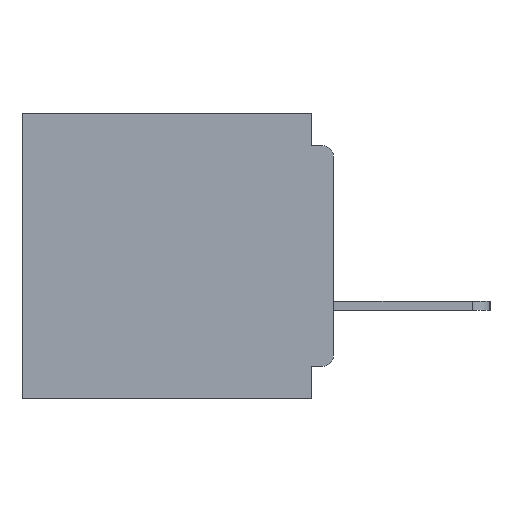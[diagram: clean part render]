
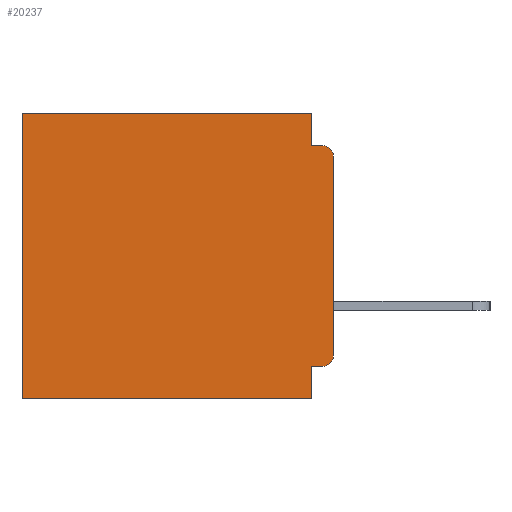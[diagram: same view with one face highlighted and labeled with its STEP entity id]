
A CAD part, left-side view. The second image highlights one B-rep face of the part: STEP entity #20237.
In plain terms, the highlighted planar face has unit normal (-1, 0, 0).
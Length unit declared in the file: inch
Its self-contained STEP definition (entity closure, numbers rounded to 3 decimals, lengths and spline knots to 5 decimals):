
#85 = EDGE_CURVE ( 'NONE', #8060, #34888, #16033, .T. ) ;
#552 = DIRECTION ( 'NONE',  ( 0., 0., -1. ) ) ;
#798 = LINE ( 'NONE', #12453, #29090 ) ;
#1566 = VECTOR ( 'NONE', #15510, 39.37008 ) ;
#2471 = LINE ( 'NONE', #6674, #1566 ) ;
#4278 = CIRCLE ( 'NONE', #12741, 0.015 ) ;
#5856 = VECTOR ( 'NONE', #15302, 39.37008 ) ;
#5936 = CARTESIAN_POINT ( 'NONE',  ( 0.3, 0.437, -0.4 ) ) ;
#6674 = CARTESIAN_POINT ( 'NONE',  ( 0.3, 0., -0.4 ) ) ;
#6757 = LINE ( 'NONE', #26754, #5856 ) ;
#6865 = EDGE_LOOP ( 'NONE', ( #32258, #36912, #10591, #34715, #27442, #28872, #13119, #13821, #22444, #24049 ) ) ;
#7541 = VECTOR ( 'NONE', #28860, 39.37008 ) ;
#8060 = VERTEX_POINT ( 'NONE', #28164 ) ;
#8603 = CARTESIAN_POINT ( 'NONE',  ( 0.3, 0., 0. ) ) ;
#8716 = VERTEX_POINT ( 'NONE', #36940 ) ;
#8830 = EDGE_CURVE ( 'NONE', #34888, #22767, #23055, .T. ) ;
#9380 = DIRECTION ( 'NONE',  ( -1., 0., 0. ) ) ;
#9565 = EDGE_CURVE ( 'NONE', #21125, #27947, #4278, .T. ) ;
#10591 = ORIENTED_EDGE ( 'NONE', *, *, #8830, .F. ) ;
#10648 = VERTEX_POINT ( 'NONE', #20290 ) ;
#11104 = AXIS2_PLACEMENT_3D ( 'NONE', #16122, #36418, #19106 ) ;
#12453 = CARTESIAN_POINT ( 'NONE',  ( 0.3, 0., -0.4 ) ) ;
#12727 = CARTESIAN_POINT ( 'NONE',  ( 0.3, 0.031, -0.045 ) ) ;
#12741 = AXIS2_PLACEMENT_3D ( 'NONE', #35406, #18072, #552 ) ;
#13091 = CARTESIAN_POINT ( 'NONE',  ( 0.3, 0.437, 0. ) ) ;
#13119 = ORIENTED_EDGE ( 'NONE', *, *, #14082, .F. ) ;
#13821 = ORIENTED_EDGE ( 'NONE', *, *, #21458, .F. ) ;
#14082 = EDGE_CURVE ( 'NONE', #23741, #10648, #798, .T. ) ;
#14494 = VECTOR ( 'NONE', #23572, 39.37008 ) ;
#15226 = AXIS2_PLACEMENT_3D ( 'NONE', #26861, #9380, #29796 ) ;
#15302 = DIRECTION ( 'NONE',  ( 0., 1., 0. ) ) ;
#15510 = DIRECTION ( 'NONE',  ( 0., 0., -1. ) ) ;
#16033 = LINE ( 'NONE', #19001, #37380 ) ;
#16122 = CARTESIAN_POINT ( 'NONE',  ( 0.3, 0., -0.4 ) ) ;
#18072 = DIRECTION ( 'NONE',  ( -1., 0., 0. ) ) ;
#18579 = CARTESIAN_POINT ( 'NONE',  ( 0.3, 0.015, -0.045 ) ) ;
#18784 = DIRECTION ( 'NONE',  ( 0., 0., -1. ) ) ;
#19001 = CARTESIAN_POINT ( 'NONE',  ( 0.3, 0.031, 0. ) ) ;
#19106 = DIRECTION ( 'NONE',  ( 0., 0., -1. ) ) ;
#19417 = EDGE_CURVE ( 'NONE', #8716, #22767, #19707, .T. ) ;
#19707 = CIRCLE ( 'NONE', #15226, 0.015 ) ;
#20237 = ADVANCED_FACE ( 'NONE', ( #35023 ), #30620, .F. ) ;
#20290 = CARTESIAN_POINT ( 'NONE',  ( 0.3, 0.437, -0.4 ) ) ;
#20398 = DIRECTION ( 'NONE',  ( 0., 1., 0. ) ) ;
#21125 = VERTEX_POINT ( 'NONE', #21966 ) ;
#21458 = EDGE_CURVE ( 'NONE', #30169, #23741, #22239, .T. ) ;
#21966 = CARTESIAN_POINT ( 'NONE',  ( 0.3, 0.015, -0.355 ) ) ;
#22239 = LINE ( 'NONE', #35104, #14494 ) ;
#22444 = ORIENTED_EDGE ( 'NONE', *, *, #23269, .F. ) ;
#22767 = VERTEX_POINT ( 'NONE', #18579 ) ;
#23055 = LINE ( 'NONE', #25786, #7541 ) ;
#23269 = EDGE_CURVE ( 'NONE', #21125, #30169, #6757, .T. ) ;
#23572 = DIRECTION ( 'NONE',  ( 0., 0., -1. ) ) ;
#23741 = VERTEX_POINT ( 'NONE', #30857 ) ;
#24049 = ORIENTED_EDGE ( 'NONE', *, *, #9565, .T. ) ;
#25697 = LINE ( 'NONE', #5936, #26599 ) ;
#25786 = CARTESIAN_POINT ( 'NONE',  ( 0.3, 0., -0.045 ) ) ;
#26343 = DIRECTION ( 'NONE',  ( 0., 0., -1. ) ) ;
#26439 = EDGE_CURVE ( 'NONE', #8716, #27947, #2471, .T. ) ;
#26566 = VERTEX_POINT ( 'NONE', #13091 ) ;
#26599 = VECTOR ( 'NONE', #26343, 39.37008 ) ;
#26754 = CARTESIAN_POINT ( 'NONE',  ( 0.3, 0., -0.355 ) ) ;
#26861 = CARTESIAN_POINT ( 'NONE',  ( 0.3, 0.015, -0.06 ) ) ;
#27442 = ORIENTED_EDGE ( 'NONE', *, *, #31401, .T. ) ;
#27947 = VERTEX_POINT ( 'NONE', #28275 ) ;
#28164 = CARTESIAN_POINT ( 'NONE',  ( 0.3, 0.031, 0. ) ) ;
#28275 = CARTESIAN_POINT ( 'NONE',  ( 0.3, 0., -0.34 ) ) ;
#28860 = DIRECTION ( 'NONE',  ( 0., -1., 0. ) ) ;
#28872 = ORIENTED_EDGE ( 'NONE', *, *, #34654, .T. ) ;
#29090 = VECTOR ( 'NONE', #35653, 39.37008 ) ;
#29168 = VECTOR ( 'NONE', #20398, 39.37008 ) ;
#29796 = DIRECTION ( 'NONE',  ( 0., 0., -1. ) ) ;
#30169 = VERTEX_POINT ( 'NONE', #31392 ) ;
#30620 = PLANE ( 'NONE',  #11104 ) ;
#30857 = CARTESIAN_POINT ( 'NONE',  ( 0.3, 0.031, -0.4 ) ) ;
#31392 = CARTESIAN_POINT ( 'NONE',  ( 0.3, 0.031, -0.355 ) ) ;
#31401 = EDGE_CURVE ( 'NONE', #8060, #26566, #36850, .T. ) ;
#32258 = ORIENTED_EDGE ( 'NONE', *, *, #26439, .F. ) ;
#34654 = EDGE_CURVE ( 'NONE', #26566, #10648, #25697, .T. ) ;
#34715 = ORIENTED_EDGE ( 'NONE', *, *, #85, .F. ) ;
#34888 = VERTEX_POINT ( 'NONE', #12727 ) ;
#35023 = FACE_OUTER_BOUND ( 'NONE', #6865, .T. ) ;
#35104 = CARTESIAN_POINT ( 'NONE',  ( 0.3, 0.031, -0.4 ) ) ;
#35406 = CARTESIAN_POINT ( 'NONE',  ( 0.3, 0.015, -0.34 ) ) ;
#35653 = DIRECTION ( 'NONE',  ( 0., 1., 0. ) ) ;
#36418 = DIRECTION ( 'NONE',  ( 1., 0., 0. ) ) ;
#36850 = LINE ( 'NONE', #8603, #29168 ) ;
#36912 = ORIENTED_EDGE ( 'NONE', *, *, #19417, .T. ) ;
#36940 = CARTESIAN_POINT ( 'NONE',  ( 0.3, 0., -0.06 ) ) ;
#37380 = VECTOR ( 'NONE', #18784, 39.37008 ) ;
